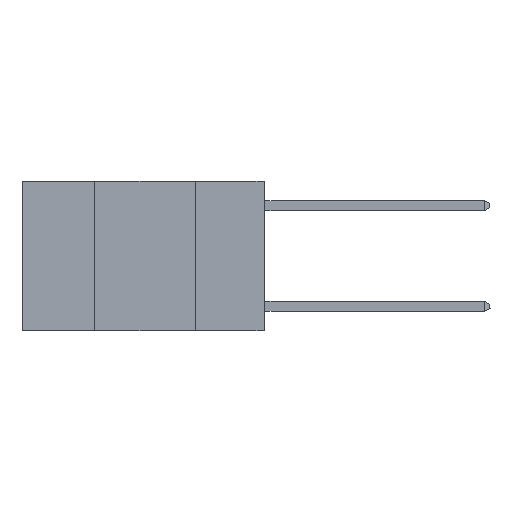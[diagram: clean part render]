
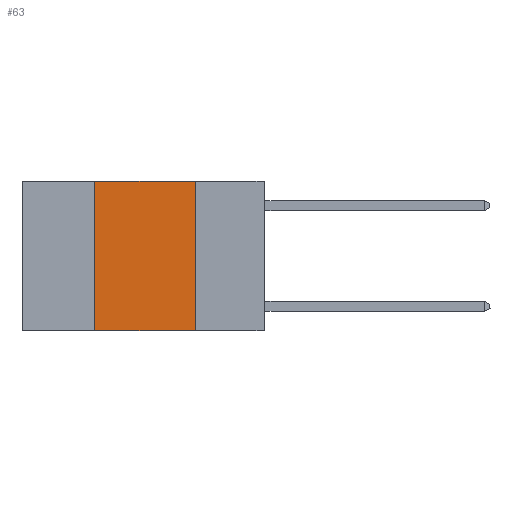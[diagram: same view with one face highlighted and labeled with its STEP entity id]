
A CAD part, left-side view. The second image highlights one B-rep face of the part: STEP entity #63.
In plain terms, the highlighted planar face has unit normal (-1, 0, 0).
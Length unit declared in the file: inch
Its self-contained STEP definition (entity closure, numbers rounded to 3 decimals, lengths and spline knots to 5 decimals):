
#63 = ADVANCED_FACE ( 'NONE', ( #23927 ), #26379, .F. ) ;
#770 = VERTEX_POINT ( 'NONE', #25505 ) ;
#890 = LINE ( 'NONE', #19588, #8220 ) ;
#1428 = ORIENTED_EDGE ( 'NONE', *, *, #21779, .F. ) ;
#2527 = CARTESIAN_POINT ( 'NONE',  ( 0., 0.17, 0. ) ) ;
#2965 = VERTEX_POINT ( 'NONE', #17719 ) ;
#3329 = CARTESIAN_POINT ( 'NONE',  ( 0., 0.6, -0.37 ) ) ;
#5207 = DIRECTION ( 'NONE',  ( 1., 0., 0. ) ) ;
#5243 = CARTESIAN_POINT ( 'NONE',  ( 0., 0.6, 0. ) ) ;
#7178 = LINE ( 'NONE', #2527, #25099 ) ;
#7989 = EDGE_CURVE ( 'NONE', #26454, #2965, #890, .T. ) ;
#8220 = VECTOR ( 'NONE', #22033, 39.37008 ) ;
#8971 = EDGE_LOOP ( 'NONE', ( #22387, #1428, #25071, #14252 ) ) ;
#9728 = VECTOR ( 'NONE', #26701, 39.37008 ) ;
#10999 = LINE ( 'NONE', #5243, #12779 ) ;
#11570 = AXIS2_PLACEMENT_3D ( 'NONE', #15999, #5207, #21874 ) ;
#11927 = EDGE_CURVE ( 'NONE', #14588, #770, #7178, .T. ) ;
#12779 = VECTOR ( 'NONE', #13452, 39.37008 ) ;
#13452 = DIRECTION ( 'NONE',  ( 0., -1., 0. ) ) ;
#13633 = CARTESIAN_POINT ( 'NONE',  ( 0., 0.17, 0. ) ) ;
#14252 = ORIENTED_EDGE ( 'NONE', *, *, #21962, .T. ) ;
#14588 = VERTEX_POINT ( 'NONE', #13633 ) ;
#15999 = CARTESIAN_POINT ( 'NONE',  ( 0., 0.6, 0. ) ) ;
#17719 = CARTESIAN_POINT ( 'NONE',  ( 0., 0.42, 0. ) ) ;
#18379 = LINE ( 'NONE', #3329, #9728 ) ;
#19588 = CARTESIAN_POINT ( 'NONE',  ( 0., 0.42, 0. ) ) ;
#20533 = CARTESIAN_POINT ( 'NONE',  ( 0., 0.42, -0.37 ) ) ;
#21779 = EDGE_CURVE ( 'NONE', #2965, #14588, #10999, .T. ) ;
#21874 = DIRECTION ( 'NONE',  ( 0., 0., -1. ) ) ;
#21962 = EDGE_CURVE ( 'NONE', #26454, #770, #18379, .T. ) ;
#22033 = DIRECTION ( 'NONE',  ( 0., 0., 1. ) ) ;
#22387 = ORIENTED_EDGE ( 'NONE', *, *, #11927, .F. ) ;
#23927 = FACE_OUTER_BOUND ( 'NONE', #8971, .T. ) ;
#25071 = ORIENTED_EDGE ( 'NONE', *, *, #7989, .F. ) ;
#25099 = VECTOR ( 'NONE', #25888, 39.37008 ) ;
#25505 = CARTESIAN_POINT ( 'NONE',  ( 0., 0.17, -0.37 ) ) ;
#25888 = DIRECTION ( 'NONE',  ( 0., 0., -1. ) ) ;
#26379 = PLANE ( 'NONE',  #11570 ) ;
#26454 = VERTEX_POINT ( 'NONE', #20533 ) ;
#26701 = DIRECTION ( 'NONE',  ( 0., -1., 0. ) ) ;
